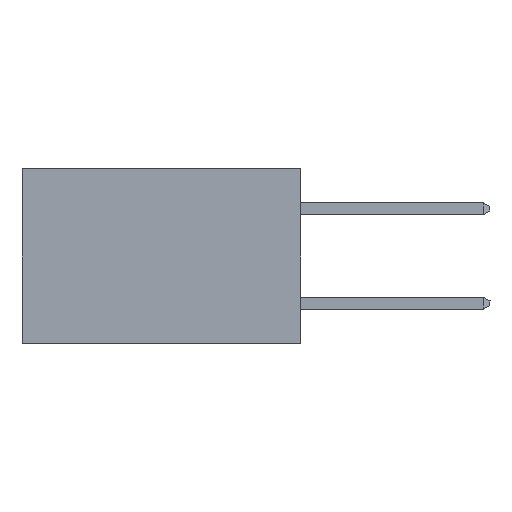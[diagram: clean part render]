
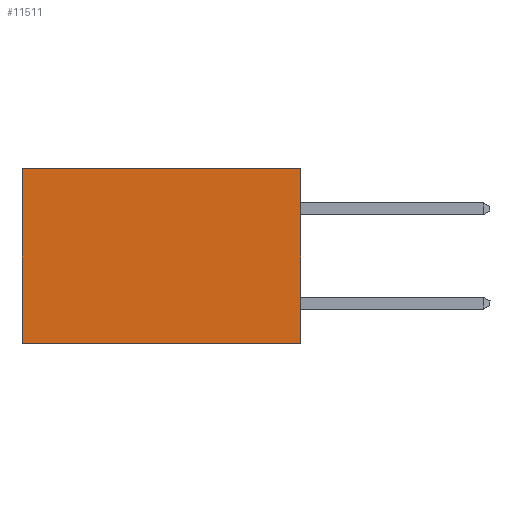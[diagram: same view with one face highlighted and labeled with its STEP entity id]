
A CAD part, left-side view. The second image highlights one B-rep face of the part: STEP entity #11511.
In plain terms, the highlighted planar face has unit normal (-1, 0, 0).
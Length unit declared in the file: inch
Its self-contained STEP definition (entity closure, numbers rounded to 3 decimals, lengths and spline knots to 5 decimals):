
#548 = CARTESIAN_POINT ( 'NONE',  ( 0.277, 0., -0.37 ) ) ;
#1725 = LINE ( 'NONE', #5866, #16314 ) ;
#2740 = ORIENTED_EDGE ( 'NONE', *, *, #6342, .T. ) ;
#3615 = VECTOR ( 'NONE', #21380, 39.37008 ) ;
#4798 = EDGE_CURVE ( 'NONE', #20449, #12749, #18090, .T. ) ;
#5434 = ORIENTED_EDGE ( 'NONE', *, *, #4798, .F. ) ;
#5703 = CARTESIAN_POINT ( 'NONE',  ( 0.277, 0.59, -0.37 ) ) ;
#5866 = CARTESIAN_POINT ( 'NONE',  ( 0.277, 0., -0.37 ) ) ;
#6327 = PLANE ( 'NONE',  #21587 ) ;
#6342 = EDGE_CURVE ( 'NONE', #6715, #19959, #18014, .T. ) ;
#6523 = ORIENTED_EDGE ( 'NONE', *, *, #7235, .F. ) ;
#6715 = VERTEX_POINT ( 'NONE', #10064 ) ;
#7234 = CARTESIAN_POINT ( 'NONE',  ( 0.277, 0., 0. ) ) ;
#7235 = EDGE_CURVE ( 'NONE', #6715, #20449, #1725, .T. ) ;
#7313 = DIRECTION ( 'NONE',  ( 0., 1., 0. ) ) ;
#9948 = DIRECTION ( 'NONE',  ( 0., 0., -1. ) ) ;
#10064 = CARTESIAN_POINT ( 'NONE',  ( 0.277, 0., 0. ) ) ;
#10357 = ORIENTED_EDGE ( 'NONE', *, *, #12526, .T. ) ;
#10381 = CARTESIAN_POINT ( 'NONE',  ( 0.277, 0.59, 0. ) ) ;
#11511 = ADVANCED_FACE ( 'NONE', ( #12181 ), #6327, .F. ) ;
#12181 = FACE_OUTER_BOUND ( 'NONE', #16567, .T. ) ;
#12526 = EDGE_CURVE ( 'NONE', #19959, #12749, #19504, .T. ) ;
#12749 = VERTEX_POINT ( 'NONE', #5703 ) ;
#13211 = VECTOR ( 'NONE', #7313, 39.37008 ) ;
#14683 = VECTOR ( 'NONE', #23154, 39.37008 ) ;
#16314 = VECTOR ( 'NONE', #22070, 39.37008 ) ;
#16567 = EDGE_LOOP ( 'NONE', ( #10357, #5434, #6523, #2740 ) ) ;
#18014 = LINE ( 'NONE', #7234, #13211 ) ;
#18090 = LINE ( 'NONE', #19611, #3615 ) ;
#18965 = CARTESIAN_POINT ( 'NONE',  ( 0.277, 0., -0.37 ) ) ;
#19504 = LINE ( 'NONE', #23081, #14683 ) ;
#19611 = CARTESIAN_POINT ( 'NONE',  ( 0.277, 0., -0.37 ) ) ;
#19959 = VERTEX_POINT ( 'NONE', #10381 ) ;
#20449 = VERTEX_POINT ( 'NONE', #548 ) ;
#20765 = DIRECTION ( 'NONE',  ( 1., 0., 0. ) ) ;
#21380 = DIRECTION ( 'NONE',  ( 0., 1., 0. ) ) ;
#21587 = AXIS2_PLACEMENT_3D ( 'NONE', #18965, #20765, #9948 ) ;
#22070 = DIRECTION ( 'NONE',  ( 0., 0., -1. ) ) ;
#23081 = CARTESIAN_POINT ( 'NONE',  ( 0.277, 0.59, -0.37 ) ) ;
#23154 = DIRECTION ( 'NONE',  ( 0., 0., -1. ) ) ;
